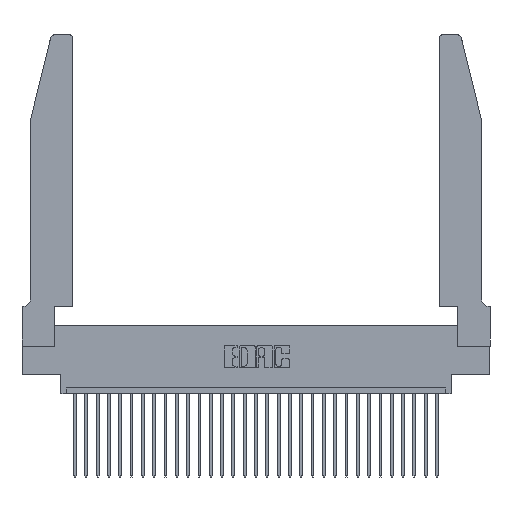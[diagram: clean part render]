
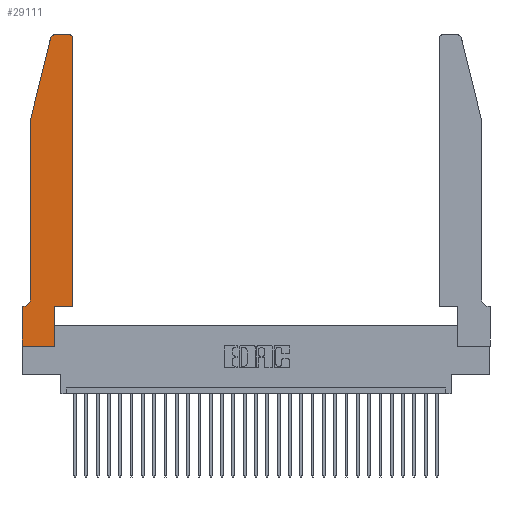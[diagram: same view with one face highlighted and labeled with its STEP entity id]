
A CAD part, top view. The second image highlights one B-rep face of the part: STEP entity #29111.
In plain terms, the highlighted planar face has unit normal (0, 0, 1).
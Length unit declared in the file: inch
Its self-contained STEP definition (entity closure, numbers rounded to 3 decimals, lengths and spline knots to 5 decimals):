
#194 = FACE_OUTER_BOUND ( 'NONE', #4813, .T. ) ;
#751 = LINE ( 'NONE', #1719, #18626 ) ;
#1067 = ORIENTED_EDGE ( 'NONE', *, *, #27989, .T. ) ;
#1102 = LINE ( 'NONE', #24072, #25734 ) ;
#1431 = AXIS2_PLACEMENT_3D ( 'NONE', #10537, #24900, #13051 ) ;
#1719 = CARTESIAN_POINT ( 'NONE',  ( 0.0755, 0.35, 0.37 ) ) ;
#1824 = CARTESIAN_POINT ( 'NONE',  ( 0.0755, 2., 0.37 ) ) ;
#2364 = LINE ( 'NONE', #11514, #16459 ) ;
#2501 = CARTESIAN_POINT ( 'NONE',  ( 0.0055, 0.35, 0.37 ) ) ;
#2698 = LINE ( 'NONE', #8724, #20200 ) ;
#3005 = EDGE_CURVE ( 'NONE', #4249, #25226, #14962, .T. ) ;
#3185 = VERTEX_POINT ( 'NONE', #11486 ) ;
#3197 = DIRECTION ( 'NONE',  ( 0., 1., 0. ) ) ;
#3416 = DIRECTION ( 'NONE',  ( -0.239, -0.971, 0. ) ) ;
#3617 = ORIENTED_EDGE ( 'NONE', *, *, #12691, .T. ) ;
#3947 = VECTOR ( 'NONE', #3197, 39.37008 ) ;
#4116 = DIRECTION ( 'NONE',  ( -1., 0., 0. ) ) ;
#4249 = VERTEX_POINT ( 'NONE', #27542 ) ;
#4442 = DIRECTION ( 'NONE',  ( 0., -1., 0. ) ) ;
#4639 = ORIENTED_EDGE ( 'NONE', *, *, #20274, .T. ) ;
#4722 = LINE ( 'NONE', #17414, #3947 ) ;
#4813 = EDGE_LOOP ( 'NONE', ( #4639, #16812, #19760, #29398, #23288, #21704, #19327, #7731, #3617, #1067, #11581, #15611 ) ) ;
#4921 = DIRECTION ( 'NONE',  ( 0., 0., 1. ) ) ;
#5843 = EDGE_CURVE ( 'NONE', #29474, #12833, #11658, .T. ) ;
#5936 = EDGE_CURVE ( 'NONE', #21996, #3185, #26626, .T. ) ;
#7201 = EDGE_CURVE ( 'NONE', #23837, #29474, #2698, .T. ) ;
#7731 = ORIENTED_EDGE ( 'NONE', *, *, #24633, .T. ) ;
#7764 = PLANE ( 'NONE',  #1431 ) ;
#8042 = EDGE_CURVE ( 'NONE', #26707, #21996, #751, .T. ) ;
#8724 = CARTESIAN_POINT ( 'NONE',  ( 0.4505, 0.35, 0.37 ) ) ;
#9680 = VECTOR ( 'NONE', #3416, 39.37008 ) ;
#10537 = CARTESIAN_POINT ( 'NONE',  ( 0., 0.35, 0.37 ) ) ;
#10775 = CARTESIAN_POINT ( 'NONE',  ( 0.4505, 0.35, 0.37 ) ) ;
#11486 = CARTESIAN_POINT ( 'NONE',  ( 0., 0., 0.37 ) ) ;
#11514 = CARTESIAN_POINT ( 'NONE',  ( 0., 0., 0.37 ) ) ;
#11581 = ORIENTED_EDGE ( 'NONE', *, *, #7201, .T. ) ;
#11583 = EDGE_CURVE ( 'NONE', #19505, #28438, #15495, .T. ) ;
#11658 = CIRCLE ( 'NONE', #23858, 0.03 ) ;
#12120 = DIRECTION ( 'NONE',  ( -1., 0., 0. ) ) ;
#12407 = VECTOR ( 'NONE', #17265, 39.37008 ) ;
#12691 = EDGE_CURVE ( 'NONE', #27505, #16857, #4722, .T. ) ;
#12833 = VERTEX_POINT ( 'NONE', #22666 ) ;
#13051 = DIRECTION ( 'NONE',  ( 1., 0., 0. ) ) ;
#13249 = AXIS2_PLACEMENT_3D ( 'NONE', #16065, #18627, #16171 ) ;
#14315 = CARTESIAN_POINT ( 'NONE',  ( 0.4205, 2.72, 0.37 ) ) ;
#14385 = LINE ( 'NONE', #10775, #29778 ) ;
#14403 = CARTESIAN_POINT ( 'NONE',  ( 0.0755, 2., 0.37 ) ) ;
#14493 = LINE ( 'NONE', #19466, #9680 ) ;
#14962 = CIRCLE ( 'NONE', #26749, 0.03 ) ;
#15495 = LINE ( 'NONE', #1824, #27158 ) ;
#15611 = ORIENTED_EDGE ( 'NONE', *, *, #5843, .T. ) ;
#16065 = CARTESIAN_POINT ( 'NONE',  ( 0.0055, 0.42, 0.37 ) ) ;
#16171 = DIRECTION ( 'NONE',  ( -1., 0., 0. ) ) ;
#16459 = VECTOR ( 'NONE', #28238, 39.37008 ) ;
#16751 = CARTESIAN_POINT ( 'NONE',  ( 0.0755, 0.42, 0.37 ) ) ;
#16812 = ORIENTED_EDGE ( 'NONE', *, *, #3005, .T. ) ;
#16857 = VERTEX_POINT ( 'NONE', #20362 ) ;
#17265 = DIRECTION ( 'NONE',  ( 0., -1., 0. ) ) ;
#17414 = CARTESIAN_POINT ( 'NONE',  ( 0.2865, 0.35, 0.37 ) ) ;
#17732 = DIRECTION ( 'NONE',  ( 0., 0., 1. ) ) ;
#18626 = VECTOR ( 'NONE', #4116, 39.37008 ) ;
#18627 = DIRECTION ( 'NONE',  ( 0., 0., -1. ) ) ;
#19327 = ORIENTED_EDGE ( 'NONE', *, *, #5936, .T. ) ;
#19466 = CARTESIAN_POINT ( 'NONE',  ( 0.0755, 2., 0.37 ) ) ;
#19505 = VERTEX_POINT ( 'NONE', #14403 ) ;
#19604 = CARTESIAN_POINT ( 'NONE',  ( 0., 0., 0.37 ) ) ;
#19625 = CIRCLE ( 'NONE', #13249, 0.07 ) ;
#19760 = ORIENTED_EDGE ( 'NONE', *, *, #19880, .T. ) ;
#19880 = EDGE_CURVE ( 'NONE', #25226, #19505, #14493, .T. ) ;
#20200 = VECTOR ( 'NONE', #20442, 39.37008 ) ;
#20274 = EDGE_CURVE ( 'NONE', #12833, #4249, #1102, .T. ) ;
#20362 = CARTESIAN_POINT ( 'NONE',  ( 0.2865, 0.35, 0.37 ) ) ;
#20442 = DIRECTION ( 'NONE',  ( 0., 1., 0. ) ) ;
#20524 = DIRECTION ( 'NONE',  ( 1., 0., 0. ) ) ;
#21704 = ORIENTED_EDGE ( 'NONE', *, *, #8042, .T. ) ;
#21996 = VERTEX_POINT ( 'NONE', #28016 ) ;
#22605 = EDGE_CURVE ( 'NONE', #28438, #26707, #19625, .T. ) ;
#22666 = CARTESIAN_POINT ( 'NONE',  ( 0.4205, 2.75, 0.37 ) ) ;
#23288 = ORIENTED_EDGE ( 'NONE', *, *, #22605, .T. ) ;
#23527 = CARTESIAN_POINT ( 'NONE',  ( 0.4505, 2.72, 0.37 ) ) ;
#23837 = VERTEX_POINT ( 'NONE', #28177 ) ;
#23858 = AXIS2_PLACEMENT_3D ( 'NONE', #14315, #4921, #26273 ) ;
#24072 = CARTESIAN_POINT ( 'NONE',  ( 0.2605, 2.75, 0.37 ) ) ;
#24633 = EDGE_CURVE ( 'NONE', #3185, #27505, #2364, .T. ) ;
#24900 = DIRECTION ( 'NONE',  ( 0., 0., 1. ) ) ;
#25226 = VERTEX_POINT ( 'NONE', #28201 ) ;
#25674 = CARTESIAN_POINT ( 'NONE',  ( 0.2865, 0., 0.37 ) ) ;
#25734 = VECTOR ( 'NONE', #12120, 39.37008 ) ;
#26273 = DIRECTION ( 'NONE',  ( 1., 0., 0. ) ) ;
#26626 = LINE ( 'NONE', #19604, #12407 ) ;
#26707 = VERTEX_POINT ( 'NONE', #2501 ) ;
#26749 = AXIS2_PLACEMENT_3D ( 'NONE', #27054, #17732, #29792 ) ;
#27054 = CARTESIAN_POINT ( 'NONE',  ( 0.284, 2.72, 0.37 ) ) ;
#27158 = VECTOR ( 'NONE', #4442, 39.37008 ) ;
#27505 = VERTEX_POINT ( 'NONE', #25674 ) ;
#27542 = CARTESIAN_POINT ( 'NONE',  ( 0.284, 2.75, 0.37 ) ) ;
#27989 = EDGE_CURVE ( 'NONE', #16857, #23837, #14385, .T. ) ;
#28016 = CARTESIAN_POINT ( 'NONE',  ( 0., 0.35, 0.37 ) ) ;
#28177 = CARTESIAN_POINT ( 'NONE',  ( 0.4505, 0.35, 0.37 ) ) ;
#28201 = CARTESIAN_POINT ( 'NONE',  ( 0.25487, 2.72718, 0.37 ) ) ;
#28238 = DIRECTION ( 'NONE',  ( 1., 0., 0. ) ) ;
#28438 = VERTEX_POINT ( 'NONE', #16751 ) ;
#29111 = ADVANCED_FACE ( 'NONE', ( #194 ), #7764, .T. ) ;
#29398 = ORIENTED_EDGE ( 'NONE', *, *, #11583, .T. ) ;
#29474 = VERTEX_POINT ( 'NONE', #23527 ) ;
#29778 = VECTOR ( 'NONE', #20524, 39.37008 ) ;
#29792 = DIRECTION ( 'NONE',  ( 1., 0., 0. ) ) ;
